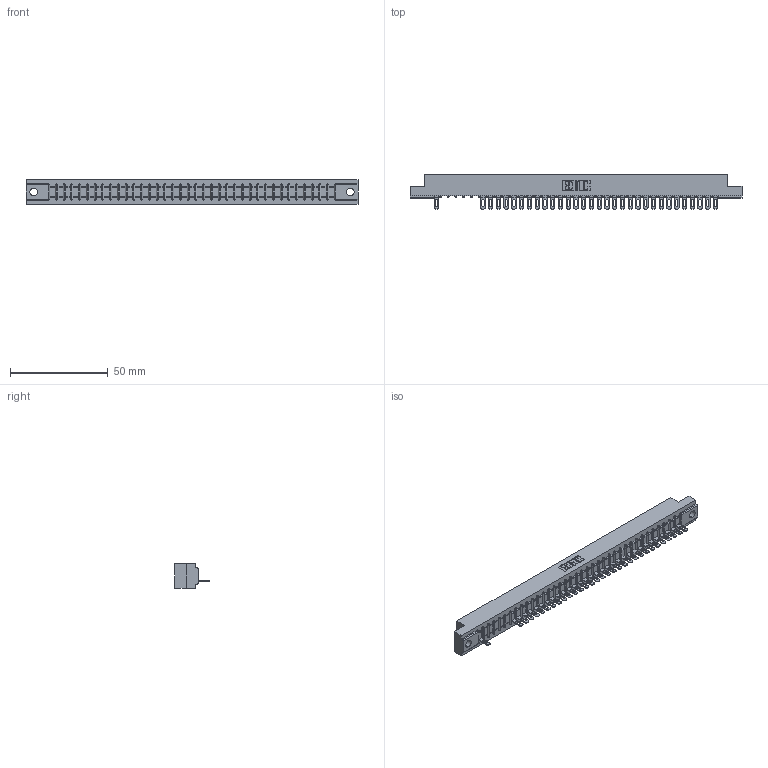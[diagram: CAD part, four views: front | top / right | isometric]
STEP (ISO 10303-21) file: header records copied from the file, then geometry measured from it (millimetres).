
FILE_DESCRIPTION (( 'STEP AP203' ), '1' );
FILE_NAME ('357-037-501-104.STEP', '2018-08-10T07:42:54', ( '' ), ( '' ), 'SwSTEP 2.0', 'SolidWorks 2016', '' );
FILE_SCHEMA (( 'CONFIG_CONTROL_DESIGN' ));
Length unit declared in the file: inch
Products named in the file (3): 307 Part_.156 Dia Mounting Holes; 307-290-002_501; 357-037-501-104
Assembly tree (33 placements, depth 2):
  357-037-501-104
    307 Part_.156 Dia Mounting Holes
    307-290-002_501  x32
Bounding box: 169.62 x 17.42 x 12.7 mm (x, y, z)
Volume: 17891.6 mm3; surface area: 21511.8 mm2
Topology: 33 solids, 33 shells, 2702 faces, 8295 edges, 5426 vertices
Faces by surface type: plane 1552, cylinder 1074, sphere 76
Entity records: 33388 total; most frequent: CARTESIAN_POINT 5657, ORIENTED_EDGE 5650, DIRECTION 5489, EDGE_CURVE 2825, LINE 2165, VECTOR 2165, VERTEX_POINT 1830, AXIS2_PLACEMENT_3D 1662
